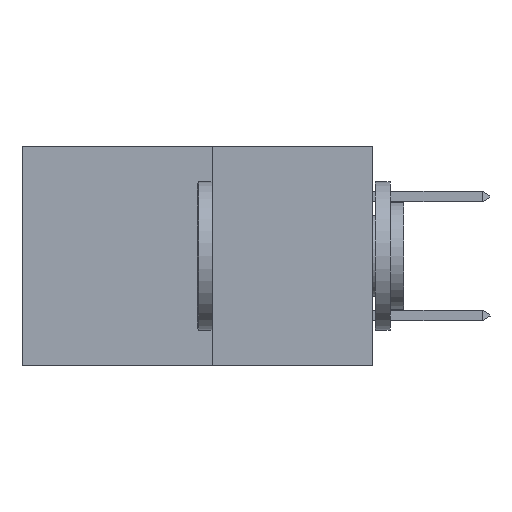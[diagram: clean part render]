
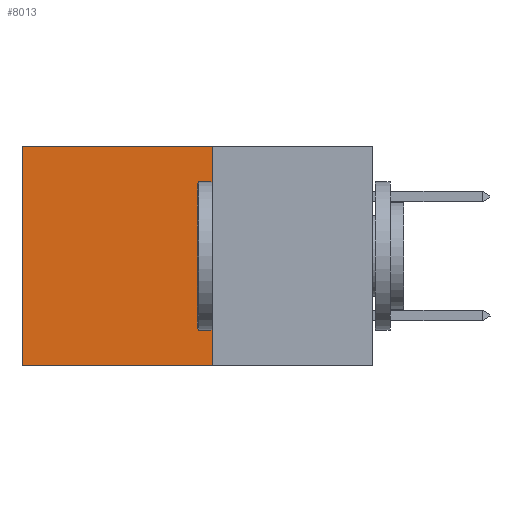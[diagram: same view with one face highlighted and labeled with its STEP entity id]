
A CAD part, left-side view. The second image highlights one B-rep face of the part: STEP entity #8013.
In plain terms, the highlighted planar face has unit normal (-1, 0, 0).
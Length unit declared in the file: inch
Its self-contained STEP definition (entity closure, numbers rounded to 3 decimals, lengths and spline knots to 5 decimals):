
#453 = VECTOR ( 'NONE', #2952, 39.37008 ) ;
#823 = CARTESIAN_POINT ( 'NONE',  ( 0.277, 0.27, -0.37 ) ) ;
#1510 = CARTESIAN_POINT ( 'NONE',  ( 0.277, 0.27, 0. ) ) ;
#1655 = ORIENTED_EDGE ( 'NONE', *, *, #2135, .T. ) ;
#1680 = CARTESIAN_POINT ( 'NONE',  ( 0.277, 0.59, -0.37 ) ) ;
#1883 = EDGE_CURVE ( 'NONE', #9313, #2536, #10023, .T. ) ;
#2135 = EDGE_CURVE ( 'NONE', #2536, #3267, #7126, .T. ) ;
#2536 = VERTEX_POINT ( 'NONE', #4442 ) ;
#2952 = DIRECTION ( 'NONE',  ( 0., 0., -1. ) ) ;
#3142 = CARTESIAN_POINT ( 'NONE',  ( 0.277, 0.27, -0.37 ) ) ;
#3267 = VERTEX_POINT ( 'NONE', #1680 ) ;
#4229 = VECTOR ( 'NONE', #9098, 39.37008 ) ;
#4442 = CARTESIAN_POINT ( 'NONE',  ( 0.277, 0.59, 0. ) ) ;
#4807 = DIRECTION ( 'NONE',  ( 1., 0., 0. ) ) ;
#4987 = CARTESIAN_POINT ( 'NONE',  ( 0.277, 0.27, -0.37 ) ) ;
#5160 = ORIENTED_EDGE ( 'NONE', *, *, #1883, .T. ) ;
#5360 = EDGE_CURVE ( 'NONE', #10577, #3267, #8402, .T. ) ;
#5782 = VECTOR ( 'NONE', #9003, 39.37008 ) ;
#5785 = DIRECTION ( 'NONE',  ( 0., 1., 0. ) ) ;
#6257 = EDGE_LOOP ( 'NONE', ( #1655, #10120, #9073, #5160 ) ) ;
#6927 = EDGE_CURVE ( 'NONE', #9313, #10577, #7634, .T. ) ;
#7126 = LINE ( 'NONE', #10377, #453 ) ;
#7166 = CARTESIAN_POINT ( 'NONE',  ( 0.277, 0.27, -0.37 ) ) ;
#7634 = LINE ( 'NONE', #823, #5782 ) ;
#8013 = ADVANCED_FACE ( 'NONE', ( #9407 ), #8740, .F. ) ;
#8155 = VECTOR ( 'NONE', #5785, 39.37008 ) ;
#8212 = CARTESIAN_POINT ( 'NONE',  ( 0.277, 0.27, 0. ) ) ;
#8402 = LINE ( 'NONE', #4987, #8155 ) ;
#8740 = PLANE ( 'NONE',  #9423 ) ;
#9003 = DIRECTION ( 'NONE',  ( 0., 0., -1. ) ) ;
#9073 = ORIENTED_EDGE ( 'NONE', *, *, #6927, .F. ) ;
#9098 = DIRECTION ( 'NONE',  ( 0., 1., 0. ) ) ;
#9313 = VERTEX_POINT ( 'NONE', #8212 ) ;
#9407 = FACE_OUTER_BOUND ( 'NONE', #6257, .T. ) ;
#9423 = AXIS2_PLACEMENT_3D ( 'NONE', #7166, #4807, #10261 ) ;
#10023 = LINE ( 'NONE', #1510, #4229 ) ;
#10120 = ORIENTED_EDGE ( 'NONE', *, *, #5360, .F. ) ;
#10261 = DIRECTION ( 'NONE',  ( 0., 0., -1. ) ) ;
#10377 = CARTESIAN_POINT ( 'NONE',  ( 0.277, 0.59, -0.37 ) ) ;
#10577 = VERTEX_POINT ( 'NONE', #3142 ) ;
